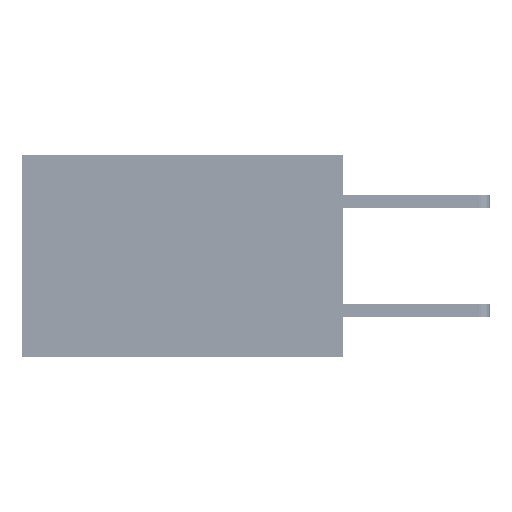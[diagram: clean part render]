
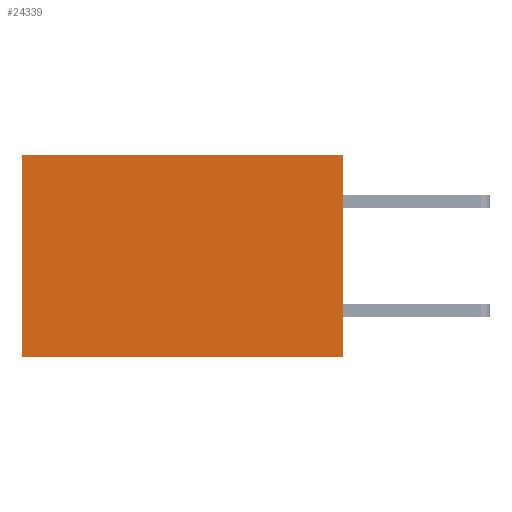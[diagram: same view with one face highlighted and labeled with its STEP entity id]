
A CAD part, left-side view. The second image highlights one B-rep face of the part: STEP entity #24339.
In plain terms, the highlighted planar face has unit normal (-1, 0, 0).
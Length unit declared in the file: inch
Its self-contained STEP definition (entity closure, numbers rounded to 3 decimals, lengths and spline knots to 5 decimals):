
#523 = VECTOR ( 'NONE', #18999, 39.37008 ) ;
#1314 = ORIENTED_EDGE ( 'NONE', *, *, #26398, .T. ) ;
#1403 = PLANE ( 'NONE',  #14413 ) ;
#2286 = LINE ( 'NONE', #20492, #29702 ) ;
#2633 = ORIENTED_EDGE ( 'NONE', *, *, #19889, .F. ) ;
#2878 = DIRECTION ( 'NONE',  ( 0., 0., -1. ) ) ;
#4329 = EDGE_CURVE ( 'NONE', #14528, #25745, #2286, .T. ) ;
#4436 = ORIENTED_EDGE ( 'NONE', *, *, #23140, .T. ) ;
#5004 = CARTESIAN_POINT ( 'NONE',  ( 0.277, 0., 0. ) ) ;
#8158 = FACE_OUTER_BOUND ( 'NONE', #23587, .T. ) ;
#9472 = DIRECTION ( 'NONE',  ( 0., 0., -1. ) ) ;
#11202 = LINE ( 'NONE', #24139, #30615 ) ;
#11278 = CARTESIAN_POINT ( 'NONE',  ( 0.277, 0., -0.37 ) ) ;
#12318 = CARTESIAN_POINT ( 'NONE',  ( 0.277, 0.59, -0.37 ) ) ;
#14413 = AXIS2_PLACEMENT_3D ( 'NONE', #20018, #25334, #9472 ) ;
#14528 = VERTEX_POINT ( 'NONE', #17158 ) ;
#15059 = DIRECTION ( 'NONE',  ( 0., 1., 0. ) ) ;
#17158 = CARTESIAN_POINT ( 'NONE',  ( 0.277, 0., -0.37 ) ) ;
#18534 = DIRECTION ( 'NONE',  ( 0., 1., 0. ) ) ;
#18999 = DIRECTION ( 'NONE',  ( 0., 0., -1. ) ) ;
#19889 = EDGE_CURVE ( 'NONE', #33852, #14528, #28753, .T. ) ;
#20018 = CARTESIAN_POINT ( 'NONE',  ( 0.277, 0., -0.37 ) ) ;
#20492 = CARTESIAN_POINT ( 'NONE',  ( 0.277, 0., -0.37 ) ) ;
#21354 = VECTOR ( 'NONE', #15059, 39.37008 ) ;
#23140 = EDGE_CURVE ( 'NONE', #33736, #25745, #11202, .T. ) ;
#23314 = ORIENTED_EDGE ( 'NONE', *, *, #4329, .F. ) ;
#23587 = EDGE_LOOP ( 'NONE', ( #4436, #23314, #2633, #1314 ) ) ;
#24139 = CARTESIAN_POINT ( 'NONE',  ( 0.277, 0.59, -0.37 ) ) ;
#24339 = ADVANCED_FACE ( 'NONE', ( #8158 ), #1403, .F. ) ;
#25334 = DIRECTION ( 'NONE',  ( 1., 0., 0. ) ) ;
#25660 = CARTESIAN_POINT ( 'NONE',  ( 0.277, 0.59, 0. ) ) ;
#25745 = VERTEX_POINT ( 'NONE', #12318 ) ;
#26398 = EDGE_CURVE ( 'NONE', #33852, #33736, #29220, .T. ) ;
#28753 = LINE ( 'NONE', #11278, #523 ) ;
#29220 = LINE ( 'NONE', #33489, #21354 ) ;
#29702 = VECTOR ( 'NONE', #18534, 39.37008 ) ;
#30615 = VECTOR ( 'NONE', #2878, 39.37008 ) ;
#33489 = CARTESIAN_POINT ( 'NONE',  ( 0.277, 0., 0. ) ) ;
#33736 = VERTEX_POINT ( 'NONE', #25660 ) ;
#33852 = VERTEX_POINT ( 'NONE', #5004 ) ;
